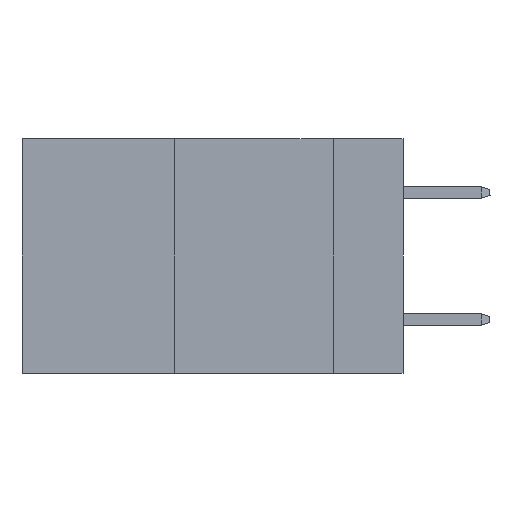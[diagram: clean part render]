
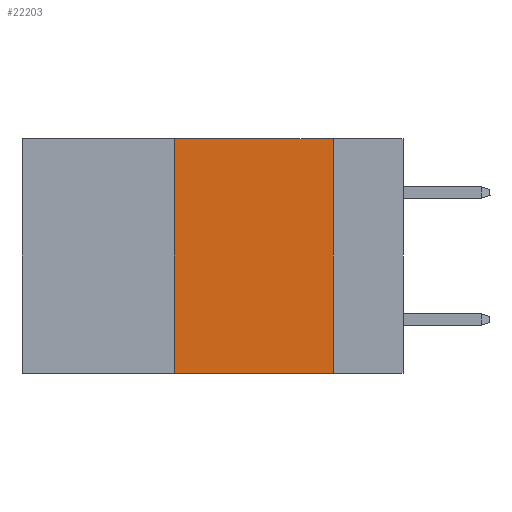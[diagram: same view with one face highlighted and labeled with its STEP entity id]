
A CAD part, left-side view. The second image highlights one B-rep face of the part: STEP entity #22203.
In plain terms, the highlighted planar face has unit normal (-1, 0, 0).
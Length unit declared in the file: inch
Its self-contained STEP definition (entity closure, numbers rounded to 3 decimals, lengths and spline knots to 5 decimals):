
#320 = LINE ( 'NONE', #27289, #12344 ) ;
#417 = LINE ( 'NONE', #10871, #5266 ) ;
#2466 = EDGE_LOOP ( 'NONE', ( #4336, #20140, #2522, #34312 ) ) ;
#2522 = ORIENTED_EDGE ( 'NONE', *, *, #30246, .F. ) ;
#2940 = FACE_OUTER_BOUND ( 'NONE', #2466, .T. ) ;
#3037 = CARTESIAN_POINT ( 'NONE',  ( 0., 0.36, 0. ) ) ;
#4108 = AXIS2_PLACEMENT_3D ( 'NONE', #19277, #16797, #29746 ) ;
#4336 = ORIENTED_EDGE ( 'NONE', *, *, #15209, .F. ) ;
#5266 = VECTOR ( 'NONE', #16767, 39.37008 ) ;
#5766 = EDGE_CURVE ( 'NONE', #32244, #21769, #417, .T. ) ;
#6901 = LINE ( 'NONE', #23262, #11257 ) ;
#7546 = CARTESIAN_POINT ( 'NONE',  ( 0., 0.11, 0. ) ) ;
#7906 = VERTEX_POINT ( 'NONE', #3037 ) ;
#10871 = CARTESIAN_POINT ( 'NONE',  ( 0., 0.6, -0.37 ) ) ;
#10914 = PLANE ( 'NONE',  #4108 ) ;
#11257 = VECTOR ( 'NONE', #25558, 39.37008 ) ;
#12344 = VECTOR ( 'NONE', #19127, 39.37008 ) ;
#15209 = EDGE_CURVE ( 'NONE', #20637, #21769, #29032, .T. ) ;
#15442 = CARTESIAN_POINT ( 'NONE',  ( 0., 0.11, -0.37 ) ) ;
#16767 = DIRECTION ( 'NONE',  ( 0., -1., 0. ) ) ;
#16797 = DIRECTION ( 'NONE',  ( 1., 0., 0. ) ) ;
#19109 = VECTOR ( 'NONE', #29210, 39.37008 ) ;
#19127 = DIRECTION ( 'NONE',  ( 0., 0., 1. ) ) ;
#19277 = CARTESIAN_POINT ( 'NONE',  ( 0., 0.6, 0. ) ) ;
#20140 = ORIENTED_EDGE ( 'NONE', *, *, #28149, .F. ) ;
#20637 = VERTEX_POINT ( 'NONE', #21478 ) ;
#21478 = CARTESIAN_POINT ( 'NONE',  ( 0., 0.11, 0. ) ) ;
#21769 = VERTEX_POINT ( 'NONE', #15442 ) ;
#22203 = ADVANCED_FACE ( 'NONE', ( #2940 ), #10914, .F. ) ;
#23262 = CARTESIAN_POINT ( 'NONE',  ( 0., 0.6, 0. ) ) ;
#25558 = DIRECTION ( 'NONE',  ( 0., -1., 0. ) ) ;
#27289 = CARTESIAN_POINT ( 'NONE',  ( 0., 0.36, 0. ) ) ;
#28149 = EDGE_CURVE ( 'NONE', #7906, #20637, #6901, .T. ) ;
#29032 = LINE ( 'NONE', #7546, #19109 ) ;
#29210 = DIRECTION ( 'NONE',  ( 0., 0., -1. ) ) ;
#29746 = DIRECTION ( 'NONE',  ( 0., 0., -1. ) ) ;
#30246 = EDGE_CURVE ( 'NONE', #32244, #7906, #320, .T. ) ;
#31213 = CARTESIAN_POINT ( 'NONE',  ( 0., 0.36, -0.37 ) ) ;
#32244 = VERTEX_POINT ( 'NONE', #31213 ) ;
#34312 = ORIENTED_EDGE ( 'NONE', *, *, #5766, .T. ) ;
